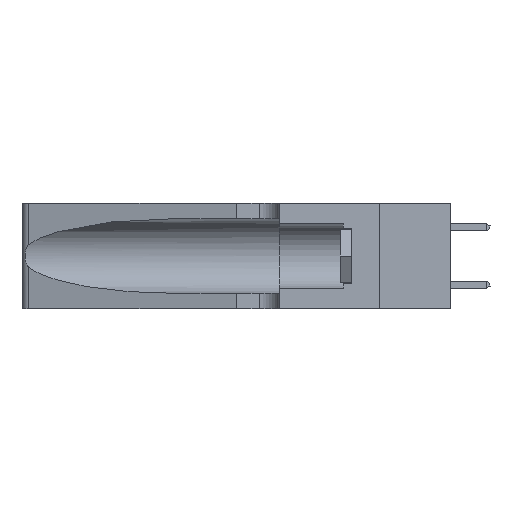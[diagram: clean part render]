
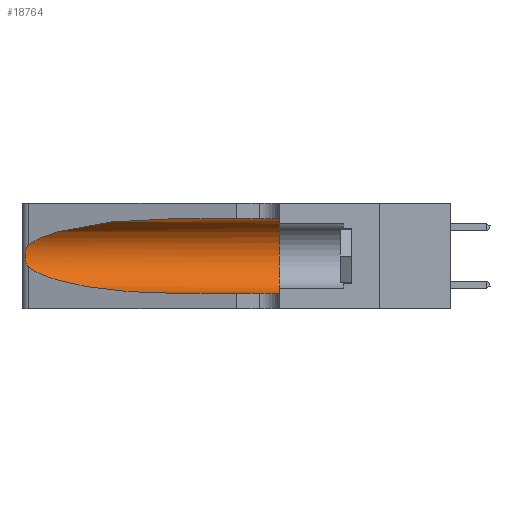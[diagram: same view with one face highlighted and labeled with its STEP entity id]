
A CAD part, left-side view. The second image highlights one B-rep face of the part: STEP entity #18764.
In plain terms, the highlighted cylindrical face has radius 3.308 mm (diameter 6.617 mm), a partial arc.
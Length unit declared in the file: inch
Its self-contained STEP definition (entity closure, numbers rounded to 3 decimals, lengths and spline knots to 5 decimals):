
#713 = AXIS2_PLACEMENT_3D ( 'NONE', #4076, #2600, #10515 ) ;
#1127 = ORIENTED_EDGE ( 'NONE', *, *, #19772, .T. ) ;
#2087 = ORIENTED_EDGE ( 'NONE', *, *, #17135, .F. ) ;
#2476 = VERTEX_POINT ( 'NONE', #24618 ) ;
#2523 = CARTESIAN_POINT ( 'NONE',  ( 0.1305, 0.72297, 0.05475 ) ) ;
#2600 = DIRECTION ( 'NONE',  ( 0., -1., 0. ) ) ;
#2666 = CARTESIAN_POINT ( 'NONE',  ( 0.1305, 1.61858, 0.31525 ) ) ;
#2714 = CARTESIAN_POINT ( 'NONE',  ( 0.26017, 1.23833, 0.17102 ) ) ;
#2851 = ORIENTED_EDGE ( 'NONE', *, *, #10054, .T. ) ;
#3764 = CARTESIAN_POINT ( 'NONE',  ( 0.2373, 1.15595, 0.28018 ) ) ;
#4040 = EDGE_CURVE ( 'NONE', #20259, #15132, #25272, .T. ) ;
#4076 = CARTESIAN_POINT ( 'NONE',  ( 0.1305, 1.61858, 0.185 ) ) ;
#4792 = CARTESIAN_POINT ( 'NONE',  ( 0.25639, 1.23184, 0.21858 ) ) ;
#4875 = LINE ( 'NONE', #2666, #6109 ) ;
#4973 = CARTESIAN_POINT ( 'NONE',  ( 0.25789, 1.23486, 0.15765 ) ) ;
#5103 = CARTESIAN_POINT ( 'NONE',  ( 0.25487, 1.22718, 0.22369 ) ) ;
#5420 = VERTEX_POINT ( 'NONE', #11173 ) ;
#5742 = EDGE_LOOP ( 'NONE', ( #18349, #2851, #19318, #1127, #15442, #2087 ) ) ;
#6109 = VECTOR ( 'NONE', #16651, 39.37008 ) ;
#6308 = CARTESIAN_POINT ( 'NONE',  ( 0.2373, 1.15595, 0.08982 ) ) ;
#7992 = B_SPLINE_CURVE_WITH_KNOTS ( 'NONE', 3,
 ( #22593, #10824, #4792, #8817, #20492, #8566, #24393, #24484, #2714, #16365, #4973, #8734, #22511, #24218 ),
 .UNSPECIFIED., .F., .F.,
 ( 4, 2, 2, 2, 2, 2, 4 ),
 ( 0., 0.00027, 0.00053, 0.00107, 0.0016, 0.00187, 0.00214 ),
 .UNSPECIFIED. ) ;
#8296 = CARTESIAN_POINT ( 'NONE',  ( 0.1305, 0.72297, 0.31525 ) ) ;
#8566 = CARTESIAN_POINT ( 'NONE',  ( 0.26018, 1.23835, 0.19895 ) ) ;
#8734 = CARTESIAN_POINT ( 'NONE',  ( 0.25639, 1.23186, 0.15144 ) ) ;
#8757 = CYLINDRICAL_SURFACE ( 'NONE', #713, 0.13025 ) ;
#8770 = DIRECTION ( 'NONE',  ( 0., 1., 0. ) ) ;
#8817 = CARTESIAN_POINT ( 'NONE',  ( 0.25787, 1.23484, 0.2124 ) ) ;
#9039 = DIRECTION ( 'NONE',  ( 0., 0., 1. ) ) ;
#10054 = EDGE_CURVE ( 'NONE', #16176, #20603, #7992, .T. ) ;
#10513 = CARTESIAN_POINT ( 'NONE',  ( 0.18966, 0.96281, 0.05475 ) ) ;
#10515 = DIRECTION ( 'NONE',  ( 0., 0., -1. ) ) ;
#10599 = CARTESIAN_POINT ( 'NONE',  ( 0.1305, 0.35, 0.185 ) ) ;
#10613 = LINE ( 'NONE', #25285, #21029 ) ;
#10824 = CARTESIAN_POINT ( 'NONE',  ( 0.25555, 1.22994, 0.2215 ) ) ;
#11047 = EDGE_CURVE ( 'NONE', #2476, #16176, #19002, .T. ) ;
#11173 = CARTESIAN_POINT ( 'NONE',  ( 0.1305, 0.72297, 0.05475 ) ) ;
#11661 = EDGE_CURVE ( 'NONE', #20603, #5420, #23831, .T. ) ;
#13551 = CARTESIAN_POINT ( 'NONE',  ( 0.18966, 0.96281, 0.31525 ) ) ;
#13651 = CARTESIAN_POINT ( 'NONE',  ( 0.1305, 0.35, 0.05475 ) ) ;
#14003 = FACE_OUTER_BOUND ( 'NONE', #5742, .T. ) ;
#15132 = VERTEX_POINT ( 'NONE', #13651 ) ;
#15442 = ORIENTED_EDGE ( 'NONE', *, *, #4040, .F. ) ;
#15619 = CARTESIAN_POINT ( 'NONE',  ( 0.25487, 1.22718, 0.22369 ) ) ;
#16088 = CARTESIAN_POINT ( 'NONE',  ( 0.25487, 1.22718, 0.14631 ) ) ;
#16176 = VERTEX_POINT ( 'NONE', #5103 ) ;
#16365 = CARTESIAN_POINT ( 'NONE',  ( 0.25856, 1.23593, 0.16098 ) ) ;
#16651 = DIRECTION ( 'NONE',  ( 0., -1., 0. ) ) ;
#17135 = EDGE_CURVE ( 'NONE', #2476, #20259, #4875, .T. ) ;
#18349 = ORIENTED_EDGE ( 'NONE', *, *, #11047, .T. ) ;
#18764 = ADVANCED_FACE ( 'NONE', ( #14003 ), #8757, .F. ) ;
#19002 =( BOUNDED_CURVE ( )  B_SPLINE_CURVE ( 3, ( #8296, #13551, #3764, #15619 ),
 .UNSPECIFIED., .F., .T. ) 
 B_SPLINE_CURVE_WITH_KNOTS ( ( 4, 4 ),
 ( 1.5708, 2.84003 ),
 .UNSPECIFIED. ) 
 CURVE ( )  GEOMETRIC_REPRESENTATION_ITEM ( )  RATIONAL_B_SPLINE_CURVE ( ( 1., 0.87, 0.87, 1. ) ) 
 REPRESENTATION_ITEM ( '' )  );
#19318 = ORIENTED_EDGE ( 'NONE', *, *, #11661, .T. ) ;
#19484 = DIRECTION ( 'NONE',  ( 0., -1., 0. ) ) ;
#19772 = EDGE_CURVE ( 'NONE', #5420, #15132, #10613, .T. ) ;
#20259 = VERTEX_POINT ( 'NONE', #20427 ) ;
#20427 = CARTESIAN_POINT ( 'NONE',  ( 0.1305, 0.35, 0.31525 ) ) ;
#20492 = CARTESIAN_POINT ( 'NONE',  ( 0.25854, 1.2359, 0.20912 ) ) ;
#20603 = VERTEX_POINT ( 'NONE', #22699 ) ;
#21029 = VECTOR ( 'NONE', #19484, 39.37008 ) ;
#22511 = CARTESIAN_POINT ( 'NONE',  ( 0.25555, 1.22993, 0.14849 ) ) ;
#22593 = CARTESIAN_POINT ( 'NONE',  ( 0.25487, 1.22718, 0.22369 ) ) ;
#22612 = AXIS2_PLACEMENT_3D ( 'NONE', #10599, #8770, #9039 ) ;
#22699 = CARTESIAN_POINT ( 'NONE',  ( 0.25487, 1.22718, 0.14631 ) ) ;
#23831 =( BOUNDED_CURVE ( )  B_SPLINE_CURVE ( 3, ( #16088, #6308, #10513, #2523 ),
 .UNSPECIFIED., .F., .F. ) 
 B_SPLINE_CURVE_WITH_KNOTS ( ( 4, 4 ),
 ( 3.44316, 4.71239 ),
 .UNSPECIFIED. ) 
 CURVE ( )  GEOMETRIC_REPRESENTATION_ITEM ( )  RATIONAL_B_SPLINE_CURVE ( ( 1., 0.87, 0.87, 1. ) ) 
 REPRESENTATION_ITEM ( '' )  );
#24218 = CARTESIAN_POINT ( 'NONE',  ( 0.25487, 1.22718, 0.14631 ) ) ;
#24393 = CARTESIAN_POINT ( 'NONE',  ( 0.26075, 1.23896, 0.19203 ) ) ;
#24484 = CARTESIAN_POINT ( 'NONE',  ( 0.26075, 1.23896, 0.178 ) ) ;
#24618 = CARTESIAN_POINT ( 'NONE',  ( 0.1305, 0.72297, 0.31525 ) ) ;
#25272 = CIRCLE ( 'NONE', #22612, 0.13025 ) ;
#25285 = CARTESIAN_POINT ( 'NONE',  ( 0.1305, 1.61858, 0.05475 ) ) ;
